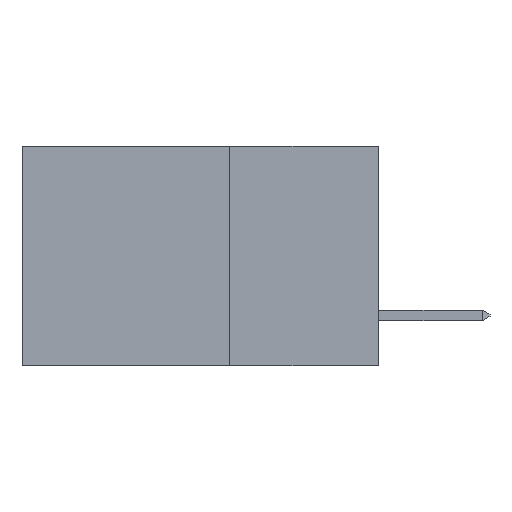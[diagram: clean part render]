
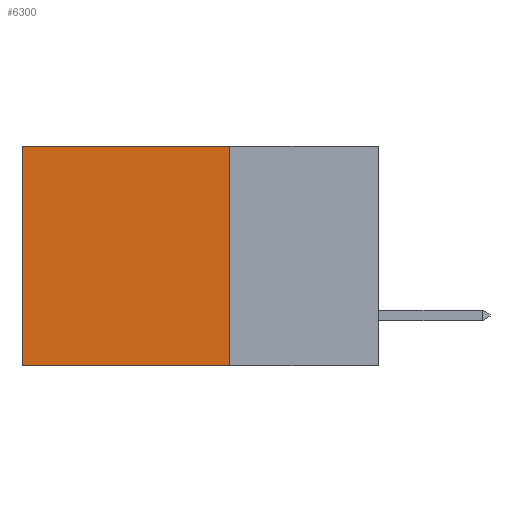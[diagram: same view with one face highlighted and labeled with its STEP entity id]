
A CAD part, left-side view. The second image highlights one B-rep face of the part: STEP entity #6300.
In plain terms, the highlighted planar face has unit normal (-1, 0, 0).
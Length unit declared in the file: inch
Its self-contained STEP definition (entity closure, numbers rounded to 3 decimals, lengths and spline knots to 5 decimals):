
#41 = DIRECTION ( 'NONE',  ( 0., 1., 0. ) ) ;
#184 = VERTEX_POINT ( 'NONE', #4243 ) ;
#235 = CARTESIAN_POINT ( 'NONE',  ( 0.2615, 0.25, -0.37 ) ) ;
#558 = AXIS2_PLACEMENT_3D ( 'NONE', #5179, #5826, #1909 ) ;
#635 = CARTESIAN_POINT ( 'NONE',  ( 0.2615, 0.6, -0.37 ) ) ;
#1212 = VECTOR ( 'NONE', #4764, 39.37008 ) ;
#1673 = CARTESIAN_POINT ( 'NONE',  ( 0.2615, 0.25, -0.37 ) ) ;
#1753 = VERTEX_POINT ( 'NONE', #635 ) ;
#1909 = DIRECTION ( 'NONE',  ( 0., 0., -1. ) ) ;
#2076 = VECTOR ( 'NONE', #3474, 39.37008 ) ;
#2604 = ORIENTED_EDGE ( 'NONE', *, *, #3205, .F. ) ;
#2976 = ORIENTED_EDGE ( 'NONE', *, *, #4790, .F. ) ;
#2994 = LINE ( 'NONE', #8038, #6264 ) ;
#3187 = VERTEX_POINT ( 'NONE', #235 ) ;
#3205 = EDGE_CURVE ( 'NONE', #3187, #1753, #5914, .T. ) ;
#3387 = EDGE_CURVE ( 'NONE', #3396, #1753, #4504, .T. ) ;
#3396 = VERTEX_POINT ( 'NONE', #5866 ) ;
#3474 = DIRECTION ( 'NONE',  ( 0., 0., -1. ) ) ;
#4243 = CARTESIAN_POINT ( 'NONE',  ( 0.2615, 0.25, 0. ) ) ;
#4504 = LINE ( 'NONE', #5295, #1212 ) ;
#4528 = PLANE ( 'NONE',  #558 ) ;
#4764 = DIRECTION ( 'NONE',  ( 0., 0., -1. ) ) ;
#4790 = EDGE_CURVE ( 'NONE', #184, #3187, #5559, .T. ) ;
#4815 = CARTESIAN_POINT ( 'NONE',  ( 0.2615, 0.25, -0.37 ) ) ;
#4901 = EDGE_CURVE ( 'NONE', #184, #3396, #2994, .T. ) ;
#5179 = CARTESIAN_POINT ( 'NONE',  ( 0.2615, 0.25, -0.37 ) ) ;
#5295 = CARTESIAN_POINT ( 'NONE',  ( 0.2615, 0.6, -0.37 ) ) ;
#5559 = LINE ( 'NONE', #4815, #2076 ) ;
#5826 = DIRECTION ( 'NONE',  ( 1., 0., 0. ) ) ;
#5866 = CARTESIAN_POINT ( 'NONE',  ( 0.2615, 0.6, 0. ) ) ;
#5914 = LINE ( 'NONE', #1673, #7407 ) ;
#6078 = DIRECTION ( 'NONE',  ( 0., 1., 0. ) ) ;
#6176 = ORIENTED_EDGE ( 'NONE', *, *, #3387, .T. ) ;
#6264 = VECTOR ( 'NONE', #6078, 39.37008 ) ;
#6300 = ADVANCED_FACE ( 'NONE', ( #6748 ), #4528, .F. ) ;
#6748 = FACE_OUTER_BOUND ( 'NONE', #7445, .T. ) ;
#7407 = VECTOR ( 'NONE', #41, 39.37008 ) ;
#7445 = EDGE_LOOP ( 'NONE', ( #6176, #2604, #2976, #8083 ) ) ;
#8038 = CARTESIAN_POINT ( 'NONE',  ( 0.2615, 0.25, 0. ) ) ;
#8083 = ORIENTED_EDGE ( 'NONE', *, *, #4901, .T. ) ;
